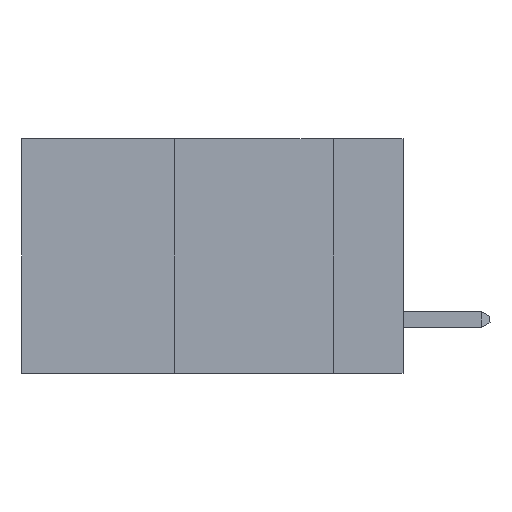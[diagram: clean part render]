
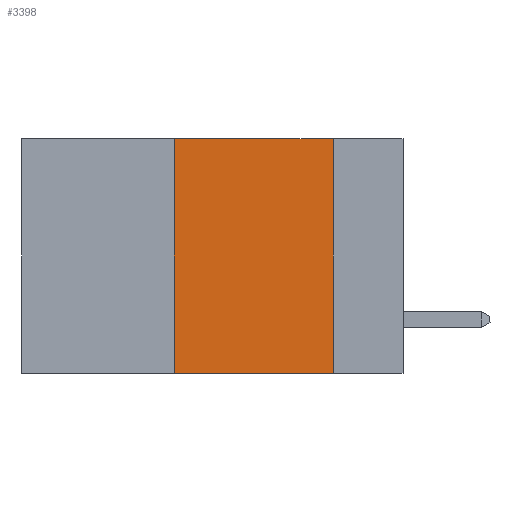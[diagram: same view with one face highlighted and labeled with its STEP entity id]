
A CAD part, left-side view. The second image highlights one B-rep face of the part: STEP entity #3398.
In plain terms, the highlighted planar face has unit normal (-1, 0, 0).
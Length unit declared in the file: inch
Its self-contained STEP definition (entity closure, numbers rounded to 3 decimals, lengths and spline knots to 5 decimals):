
#336 = ORIENTED_EDGE ( 'NONE', *, *, #18037, .T. ) ;
#610 = ORIENTED_EDGE ( 'NONE', *, *, #21578, .F. ) ;
#778 = DIRECTION ( 'NONE',  ( 1., 0., 0. ) ) ;
#1153 = CARTESIAN_POINT ( 'NONE',  ( 0., 0.6, -0.37 ) ) ;
#1356 = VECTOR ( 'NONE', #22393, 39.37008 ) ;
#1964 = ORIENTED_EDGE ( 'NONE', *, *, #13585, .F. ) ;
#2273 = FACE_OUTER_BOUND ( 'NONE', #10843, .T. ) ;
#3022 = VECTOR ( 'NONE', #10951, 39.37008 ) ;
#3104 = ORIENTED_EDGE ( 'NONE', *, *, #21550, .F. ) ;
#3398 = ADVANCED_FACE ( 'NONE', ( #2273 ), #10494, .F. ) ;
#4975 = VERTEX_POINT ( 'NONE', #7936 ) ;
#5733 = VERTEX_POINT ( 'NONE', #6157 ) ;
#6157 = CARTESIAN_POINT ( 'NONE',  ( 0., 0.11, 0. ) ) ;
#6690 = CARTESIAN_POINT ( 'NONE',  ( 0., 0.6, 0. ) ) ;
#7161 = DIRECTION ( 'NONE',  ( 0., -1., 0. ) ) ;
#7936 = CARTESIAN_POINT ( 'NONE',  ( 0., 0.11, -0.37 ) ) ;
#8318 = VECTOR ( 'NONE', #11037, 39.37008 ) ;
#9183 = AXIS2_PLACEMENT_3D ( 'NONE', #6690, #778, #14237 ) ;
#10494 = PLANE ( 'NONE',  #9183 ) ;
#10843 = EDGE_LOOP ( 'NONE', ( #1964, #610, #3104, #336 ) ) ;
#10951 = DIRECTION ( 'NONE',  ( 0., 0., 1. ) ) ;
#11037 = DIRECTION ( 'NONE',  ( 0., -1., 0. ) ) ;
#12783 = CARTESIAN_POINT ( 'NONE',  ( 0., 0.6, 0. ) ) ;
#13585 = EDGE_CURVE ( 'NONE', #5733, #4975, #16670, .T. ) ;
#14237 = DIRECTION ( 'NONE',  ( 0., 0., -1. ) ) ;
#16670 = LINE ( 'NONE', #20614, #1356 ) ;
#16894 = LINE ( 'NONE', #1153, #21211 ) ;
#18037 = EDGE_CURVE ( 'NONE', #19593, #4975, #16894, .T. ) ;
#18449 = CARTESIAN_POINT ( 'NONE',  ( 0., 0.36, 0. ) ) ;
#18628 = CARTESIAN_POINT ( 'NONE',  ( 0., 0.36, 0. ) ) ;
#18781 = CARTESIAN_POINT ( 'NONE',  ( 0., 0.36, -0.37 ) ) ;
#19593 = VERTEX_POINT ( 'NONE', #18781 ) ;
#20614 = CARTESIAN_POINT ( 'NONE',  ( 0., 0.11, 0. ) ) ;
#21211 = VECTOR ( 'NONE', #7161, 39.37008 ) ;
#21550 = EDGE_CURVE ( 'NONE', #19593, #23840, #23570, .T. ) ;
#21578 = EDGE_CURVE ( 'NONE', #23840, #5733, #22505, .T. ) ;
#22393 = DIRECTION ( 'NONE',  ( 0., 0., -1. ) ) ;
#22505 = LINE ( 'NONE', #12783, #8318 ) ;
#23570 = LINE ( 'NONE', #18449, #3022 ) ;
#23840 = VERTEX_POINT ( 'NONE', #18628 ) ;
